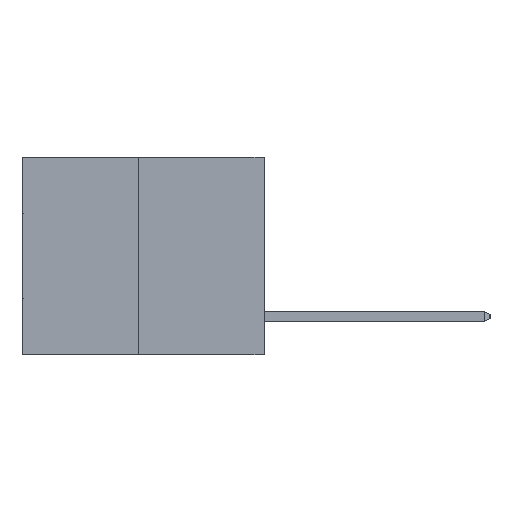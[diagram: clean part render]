
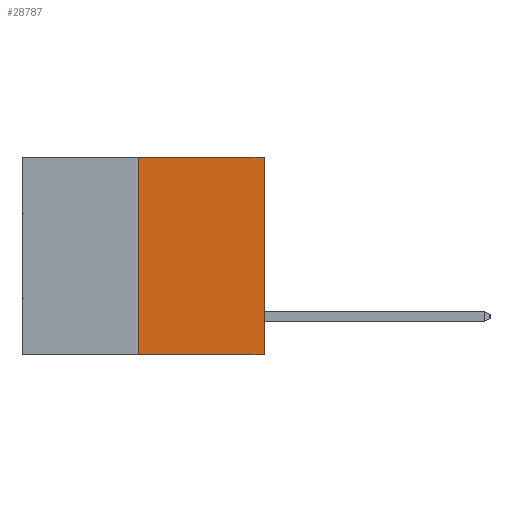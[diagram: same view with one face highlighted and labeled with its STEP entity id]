
A CAD part, left-side view. The second image highlights one B-rep face of the part: STEP entity #28787.
In plain terms, the highlighted planar face has unit normal (-1, 0, 0).
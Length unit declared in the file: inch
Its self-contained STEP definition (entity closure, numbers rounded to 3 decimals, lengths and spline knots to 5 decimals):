
#700 = VERTEX_POINT ( 'NONE', #24554 ) ;
#760 = DIRECTION ( 'NONE',  ( 1., 0., 0. ) ) ;
#958 = FACE_OUTER_BOUND ( 'NONE', #29146, .T. ) ;
#2105 = CARTESIAN_POINT ( 'NONE',  ( 0., 0.6, -0.49 ) ) ;
#3262 = AXIS2_PLACEMENT_3D ( 'NONE', #8005, #760, #14724 ) ;
#3684 = DIRECTION ( 'NONE',  ( 0., -1., 0. ) ) ;
#3851 = VECTOR ( 'NONE', #30853, 39.37008 ) ;
#7680 = LINE ( 'NONE', #27470, #13724 ) ;
#8005 = CARTESIAN_POINT ( 'NONE',  ( 0., 0.6, 0. ) ) ;
#9691 = CARTESIAN_POINT ( 'NONE',  ( 0., 0.312, 0. ) ) ;
#10933 = VECTOR ( 'NONE', #23552, 39.37008 ) ;
#12030 = LINE ( 'NONE', #31056, #10933 ) ;
#13251 = CARTESIAN_POINT ( 'NONE',  ( 0., 0.312, -0.49 ) ) ;
#13724 = VECTOR ( 'NONE', #3684, 39.37008 ) ;
#14724 = DIRECTION ( 'NONE',  ( 0., 0., -1. ) ) ;
#14886 = VERTEX_POINT ( 'NONE', #9691 ) ;
#15032 = PLANE ( 'NONE',  #3262 ) ;
#17503 = VERTEX_POINT ( 'NONE', #13251 ) ;
#17907 = ORIENTED_EDGE ( 'NONE', *, *, #27084, .F. ) ;
#18113 = EDGE_CURVE ( 'NONE', #22573, #700, #12030, .T. ) ;
#18138 = CARTESIAN_POINT ( 'NONE',  ( 0., 0., -0.49 ) ) ;
#21150 = LINE ( 'NONE', #22555, #26432 ) ;
#22555 = CARTESIAN_POINT ( 'NONE',  ( 0., 0.312, -0.49 ) ) ;
#22573 = VERTEX_POINT ( 'NONE', #18138 ) ;
#23552 = DIRECTION ( 'NONE',  ( 0., 0., 1. ) ) ;
#23873 = ORIENTED_EDGE ( 'NONE', *, *, #31001, .T. ) ;
#23964 = ORIENTED_EDGE ( 'NONE', *, *, #18113, .T. ) ;
#24554 = CARTESIAN_POINT ( 'NONE',  ( 0., 0., 0. ) ) ;
#25326 = EDGE_CURVE ( 'NONE', #14886, #700, #7680, .T. ) ;
#26432 = VECTOR ( 'NONE', #29937, 39.37008 ) ;
#27084 = EDGE_CURVE ( 'NONE', #17503, #14886, #21150, .T. ) ;
#27470 = CARTESIAN_POINT ( 'NONE',  ( 0., 0.6, 0. ) ) ;
#28336 = LINE ( 'NONE', #2105, #3851 ) ;
#28573 = ORIENTED_EDGE ( 'NONE', *, *, #25326, .F. ) ;
#28787 = ADVANCED_FACE ( 'NONE', ( #958 ), #15032, .F. ) ;
#29146 = EDGE_LOOP ( 'NONE', ( #17907, #23873, #23964, #28573 ) ) ;
#29937 = DIRECTION ( 'NONE',  ( 0., 0., 1. ) ) ;
#30853 = DIRECTION ( 'NONE',  ( 0., -1., 0. ) ) ;
#31001 = EDGE_CURVE ( 'NONE', #17503, #22573, #28336, .T. ) ;
#31056 = CARTESIAN_POINT ( 'NONE',  ( 0., 0., 0. ) ) ;
